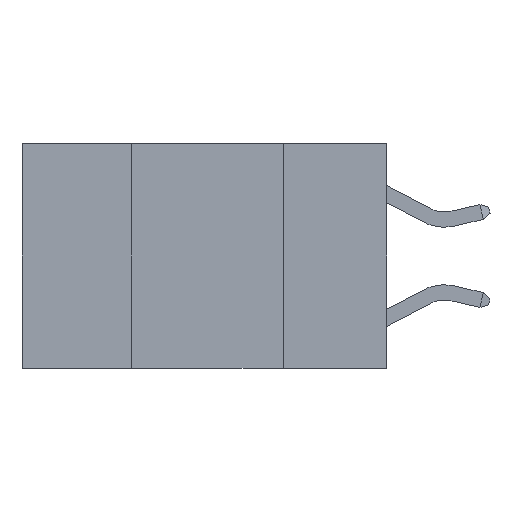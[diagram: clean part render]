
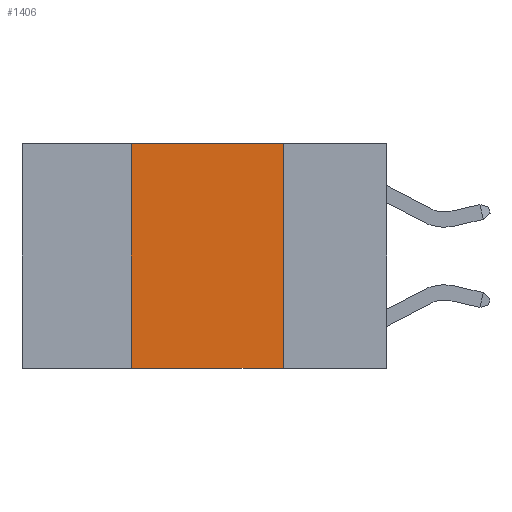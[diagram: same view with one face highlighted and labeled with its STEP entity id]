
A CAD part, left-side view. The second image highlights one B-rep face of the part: STEP entity #1406.
In plain terms, the highlighted planar face has unit normal (-1, 0, 0).
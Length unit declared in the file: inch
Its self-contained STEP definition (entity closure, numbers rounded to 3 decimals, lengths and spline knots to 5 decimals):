
#422 = CARTESIAN_POINT ( 'NONE',  ( 0., 0.17, -0.37 ) ) ;
#541 = CARTESIAN_POINT ( 'NONE',  ( 0., 0.42, 0. ) ) ;
#645 = EDGE_LOOP ( 'NONE', ( #876, #3999, #3759, #8231 ) ) ;
#876 = ORIENTED_EDGE ( 'NONE', *, *, #6649, .F. ) ;
#1003 = VECTOR ( 'NONE', #9554, 39.37008 ) ;
#1366 = VERTEX_POINT ( 'NONE', #422 ) ;
#1406 = ADVANCED_FACE ( 'NONE', ( #10324 ), #1807, .F. ) ;
#1429 = LINE ( 'NONE', #9593, #2559 ) ;
#1503 = DIRECTION ( 'NONE',  ( 0., -1., 0. ) ) ;
#1807 = PLANE ( 'NONE',  #7227 ) ;
#2501 = CARTESIAN_POINT ( 'NONE',  ( 0., 0.6, 0. ) ) ;
#2559 = VECTOR ( 'NONE', #1503, 39.37008 ) ;
#2626 = CARTESIAN_POINT ( 'NONE',  ( 0., 0.6, 0. ) ) ;
#3451 = CARTESIAN_POINT ( 'NONE',  ( 0., 0.42, -0.37 ) ) ;
#3759 = ORIENTED_EDGE ( 'NONE', *, *, #6231, .F. ) ;
#3999 = ORIENTED_EDGE ( 'NONE', *, *, #9358, .F. ) ;
#4296 = DIRECTION ( 'NONE',  ( 1., 0., 0. ) ) ;
#4350 = DIRECTION ( 'NONE',  ( 0., 0., -1. ) ) ;
#5062 = LINE ( 'NONE', #2501, #9213 ) ;
#5080 = LINE ( 'NONE', #8820, #1003 ) ;
#6231 = EDGE_CURVE ( 'NONE', #8112, #7766, #8963, .T. ) ;
#6317 = EDGE_CURVE ( 'NONE', #8112, #1366, #1429, .T. ) ;
#6627 = CARTESIAN_POINT ( 'NONE',  ( 0., 0.42, 0. ) ) ;
#6649 = EDGE_CURVE ( 'NONE', #9261, #1366, #5080, .T. ) ;
#6794 = VECTOR ( 'NONE', #9495, 39.37008 ) ;
#7227 = AXIS2_PLACEMENT_3D ( 'NONE', #2626, #4296, #4350 ) ;
#7381 = CARTESIAN_POINT ( 'NONE',  ( 0., 0.17, 0. ) ) ;
#7481 = DIRECTION ( 'NONE',  ( 0., -1., 0. ) ) ;
#7766 = VERTEX_POINT ( 'NONE', #6627 ) ;
#8112 = VERTEX_POINT ( 'NONE', #3451 ) ;
#8231 = ORIENTED_EDGE ( 'NONE', *, *, #6317, .T. ) ;
#8820 = CARTESIAN_POINT ( 'NONE',  ( 0., 0.17, 0. ) ) ;
#8963 = LINE ( 'NONE', #541, #6794 ) ;
#9213 = VECTOR ( 'NONE', #7481, 39.37008 ) ;
#9261 = VERTEX_POINT ( 'NONE', #7381 ) ;
#9358 = EDGE_CURVE ( 'NONE', #7766, #9261, #5062, .T. ) ;
#9495 = DIRECTION ( 'NONE',  ( 0., 0., 1. ) ) ;
#9554 = DIRECTION ( 'NONE',  ( 0., 0., -1. ) ) ;
#9593 = CARTESIAN_POINT ( 'NONE',  ( 0., 0.6, -0.37 ) ) ;
#10324 = FACE_OUTER_BOUND ( 'NONE', #645, .T. ) ;
